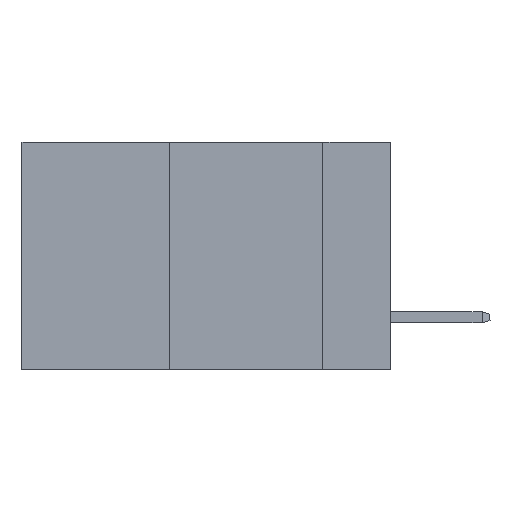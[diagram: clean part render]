
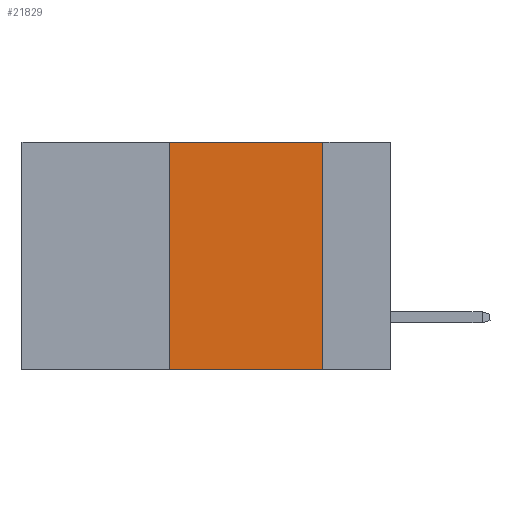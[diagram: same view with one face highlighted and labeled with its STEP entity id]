
A CAD part, left-side view. The second image highlights one B-rep face of the part: STEP entity #21829.
In plain terms, the highlighted planar face has unit normal (-1, 0, 0).
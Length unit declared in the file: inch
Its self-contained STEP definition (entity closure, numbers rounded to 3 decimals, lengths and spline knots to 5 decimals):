
#149 = EDGE_LOOP ( 'NONE', ( #15151, #11480, #11072, #22514 ) ) ;
#1336 = CARTESIAN_POINT ( 'NONE',  ( 0., 0.36, -0.37 ) ) ;
#1971 = CARTESIAN_POINT ( 'NONE',  ( 0., 0.11, 0. ) ) ;
#3959 = VECTOR ( 'NONE', #10549, 39.37008 ) ;
#4440 = VERTEX_POINT ( 'NONE', #16078 ) ;
#7599 = DIRECTION ( 'NONE',  ( 1., 0., 0. ) ) ;
#8239 = EDGE_CURVE ( 'NONE', #21578, #4440, #21059, .T. ) ;
#8269 = CARTESIAN_POINT ( 'NONE',  ( 0., 0.6, -0.37 ) ) ;
#8290 = VERTEX_POINT ( 'NONE', #8352 ) ;
#8352 = CARTESIAN_POINT ( 'NONE',  ( 0., 0.11, 0. ) ) ;
#8715 = LINE ( 'NONE', #17311, #3959 ) ;
#10060 = DIRECTION ( 'NONE',  ( 0., -1., 0. ) ) ;
#10549 = DIRECTION ( 'NONE',  ( 0., 0., 1. ) ) ;
#11072 = ORIENTED_EDGE ( 'NONE', *, *, #13194, .F. ) ;
#11211 = DIRECTION ( 'NONE',  ( 0., -1., 0. ) ) ;
#11282 = CARTESIAN_POINT ( 'NONE',  ( 0., 0.6, 0. ) ) ;
#11311 = VERTEX_POINT ( 'NONE', #21610 ) ;
#11469 = FACE_OUTER_BOUND ( 'NONE', #149, .T. ) ;
#11480 = ORIENTED_EDGE ( 'NONE', *, *, #17296, .F. ) ;
#12099 = VECTOR ( 'NONE', #10060, 39.37008 ) ;
#12452 = VECTOR ( 'NONE', #11211, 39.37008 ) ;
#12983 = LINE ( 'NONE', #11282, #12452 ) ;
#13194 = EDGE_CURVE ( 'NONE', #21578, #11311, #8715, .T. ) ;
#14727 = VECTOR ( 'NONE', #17674, 39.37008 ) ;
#15151 = ORIENTED_EDGE ( 'NONE', *, *, #15878, .F. ) ;
#15807 = LINE ( 'NONE', #1971, #14727 ) ;
#15878 = EDGE_CURVE ( 'NONE', #8290, #4440, #15807, .T. ) ;
#16078 = CARTESIAN_POINT ( 'NONE',  ( 0., 0.11, -0.37 ) ) ;
#16168 = CARTESIAN_POINT ( 'NONE',  ( 0., 0.6, 0. ) ) ;
#17296 = EDGE_CURVE ( 'NONE', #11311, #8290, #12983, .T. ) ;
#17311 = CARTESIAN_POINT ( 'NONE',  ( 0., 0.36, 0. ) ) ;
#17674 = DIRECTION ( 'NONE',  ( 0., 0., -1. ) ) ;
#19545 = DIRECTION ( 'NONE',  ( 0., 0., -1. ) ) ;
#21059 = LINE ( 'NONE', #8269, #12099 ) ;
#21168 = PLANE ( 'NONE',  #21533 ) ;
#21533 = AXIS2_PLACEMENT_3D ( 'NONE', #16168, #7599, #19545 ) ;
#21578 = VERTEX_POINT ( 'NONE', #1336 ) ;
#21610 = CARTESIAN_POINT ( 'NONE',  ( 0., 0.36, 0. ) ) ;
#21829 = ADVANCED_FACE ( 'NONE', ( #11469 ), #21168, .F. ) ;
#22514 = ORIENTED_EDGE ( 'NONE', *, *, #8239, .T. ) ;
